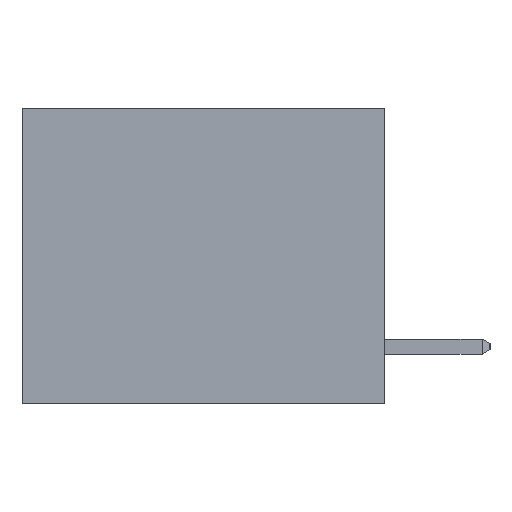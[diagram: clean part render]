
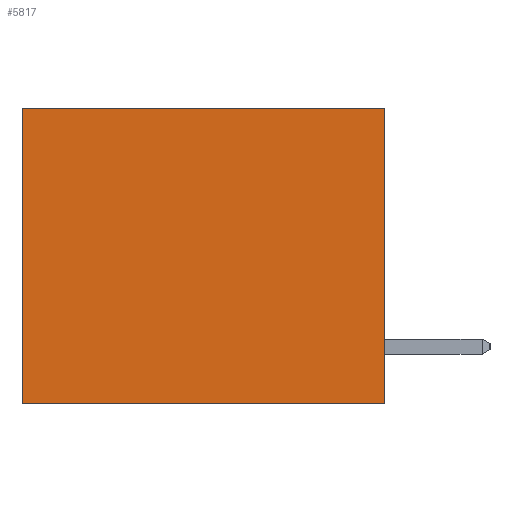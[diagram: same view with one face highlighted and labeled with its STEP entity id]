
A CAD part, left-side view. The second image highlights one B-rep face of the part: STEP entity #5817.
In plain terms, the highlighted planar face has unit normal (-1, 0, 0).
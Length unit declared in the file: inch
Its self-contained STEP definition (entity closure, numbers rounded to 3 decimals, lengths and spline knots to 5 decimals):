
#174 = LINE ( 'NONE', #17058, #14597 ) ;
#534 = CARTESIAN_POINT ( 'NONE',  ( 0.3165, 0.6, 0. ) ) ;
#1028 = CARTESIAN_POINT ( 'NONE',  ( 0.3165, 0., -0.49 ) ) ;
#1599 = EDGE_CURVE ( 'NONE', #4188, #12335, #3356, .T. ) ;
#1855 = CARTESIAN_POINT ( 'NONE',  ( 0.3165, 0.6, -0.49 ) ) ;
#2277 = LINE ( 'NONE', #1028, #12244 ) ;
#2722 = ORIENTED_EDGE ( 'NONE', *, *, #1599, .T. ) ;
#3025 = VERTEX_POINT ( 'NONE', #10725 ) ;
#3356 = LINE ( 'NONE', #3525, #11307 ) ;
#3525 = CARTESIAN_POINT ( 'NONE',  ( 0.3165, 0.6, -0.49 ) ) ;
#4188 = VERTEX_POINT ( 'NONE', #534 ) ;
#5817 = ADVANCED_FACE ( 'NONE', ( #15437 ), #15812, .F. ) ;
#6503 = ORIENTED_EDGE ( 'NONE', *, *, #15101, .F. ) ;
#6554 = EDGE_CURVE ( 'NONE', #3025, #4188, #174, .T. ) ;
#6836 = AXIS2_PLACEMENT_3D ( 'NONE', #8440, #14261, #7039 ) ;
#6942 = ORIENTED_EDGE ( 'NONE', *, *, #6554, .T. ) ;
#7039 = DIRECTION ( 'NONE',  ( 0., 0., -1. ) ) ;
#7397 = VERTEX_POINT ( 'NONE', #16387 ) ;
#8440 = CARTESIAN_POINT ( 'NONE',  ( 0.3165, 0., -0.49 ) ) ;
#9219 = DIRECTION ( 'NONE',  ( 0., 0., -1. ) ) ;
#10725 = CARTESIAN_POINT ( 'NONE',  ( 0.3165, 0., 0. ) ) ;
#10883 = DIRECTION ( 'NONE',  ( 0., 0., -1. ) ) ;
#10916 = EDGE_LOOP ( 'NONE', ( #2722, #6503, #15989, #6942 ) ) ;
#11307 = VECTOR ( 'NONE', #10883, 39.37008 ) ;
#11506 = EDGE_CURVE ( 'NONE', #3025, #7397, #13026, .T. ) ;
#12244 = VECTOR ( 'NONE', #18310, 39.37008 ) ;
#12335 = VERTEX_POINT ( 'NONE', #1855 ) ;
#13026 = LINE ( 'NONE', #13078, #18668 ) ;
#13078 = CARTESIAN_POINT ( 'NONE',  ( 0.3165, 0., -0.49 ) ) ;
#14261 = DIRECTION ( 'NONE',  ( 1., 0., 0. ) ) ;
#14597 = VECTOR ( 'NONE', #18514, 39.37008 ) ;
#15101 = EDGE_CURVE ( 'NONE', #7397, #12335, #2277, .T. ) ;
#15437 = FACE_OUTER_BOUND ( 'NONE', #10916, .T. ) ;
#15812 = PLANE ( 'NONE',  #6836 ) ;
#15989 = ORIENTED_EDGE ( 'NONE', *, *, #11506, .F. ) ;
#16387 = CARTESIAN_POINT ( 'NONE',  ( 0.3165, 0., -0.49 ) ) ;
#17058 = CARTESIAN_POINT ( 'NONE',  ( 0.3165, 0., 0. ) ) ;
#18310 = DIRECTION ( 'NONE',  ( 0., 1., 0. ) ) ;
#18514 = DIRECTION ( 'NONE',  ( 0., 1., 0. ) ) ;
#18668 = VECTOR ( 'NONE', #9219, 39.37008 ) ;
